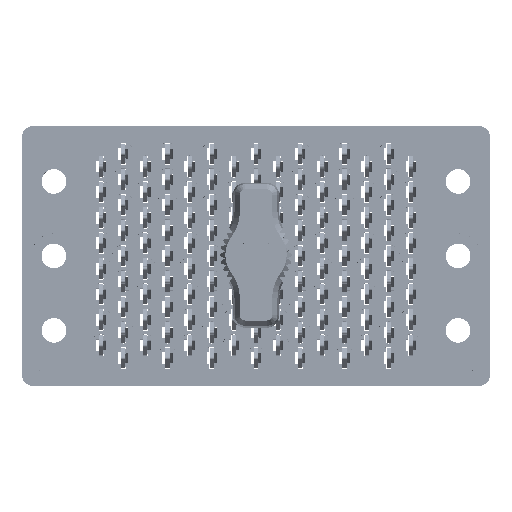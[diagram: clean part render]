
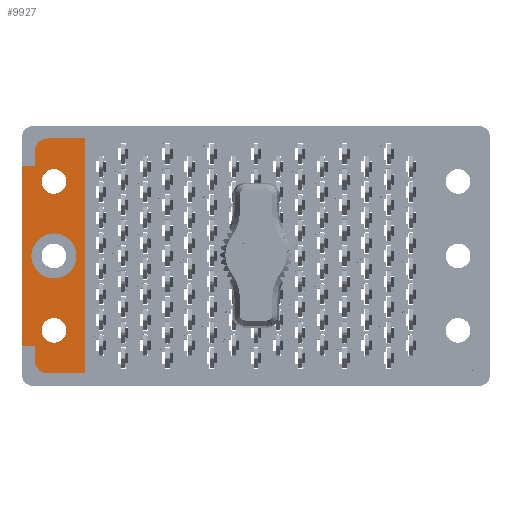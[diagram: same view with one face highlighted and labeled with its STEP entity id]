
A CAD part, top view. The second image highlights one B-rep face of the part: STEP entity #9927.
In plain terms, the highlighted planar face has unit normal (0, 0, 1).
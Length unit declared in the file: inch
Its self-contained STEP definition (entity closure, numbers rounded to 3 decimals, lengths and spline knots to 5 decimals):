
#209 = VERTEX_POINT ( 'NONE', #38791 ) ;
#692 = LINE ( 'NONE', #48378, #39513 ) ;
#1297 = AXIS2_PLACEMENT_3D ( 'NONE', #1905, #43440, #85039 ) ;
#1304 = ORIENTED_EDGE ( 'NONE', *, *, #89556, .T. ) ;
#1559 = ORIENTED_EDGE ( 'NONE', *, *, #34092, .T. ) ;
#1905 = CARTESIAN_POINT ( 'NONE',  ( -1.225, -0.615, -0.117 ) ) ;
#2947 = CARTESIAN_POINT ( 'NONE',  ( -1.3, -0.615, -0.117 ) ) ;
#5914 = EDGE_CURVE ( 'NONE', #89757, #19831, #66030, .T. ) ;
#6220 = CARTESIAN_POINT ( 'NONE',  ( -1.115, -0.4375, -0.117 ) ) ;
#6446 = EDGE_LOOP ( 'NONE', ( #1304, #7442, #56029, #1559, #35537, #18134, #103705, #23668, #94515, #49916 ) ) ;
#6774 = CIRCLE ( 'NONE', #94406, 0.1325 ) ;
#7442 = ORIENTED_EDGE ( 'NONE', *, *, #64470, .T. ) ;
#7954 = AXIS2_PLACEMENT_3D ( 'NONE', #32287, #89775, #40259 ) ;
#9914 = VERTEX_POINT ( 'NONE', #19978 ) ;
#9927 = ADVANCED_FACE ( 'NONE', ( #21981, #42694, #64714, #100878 ), #45953, .T. ) ;
#10055 = CIRCLE ( 'NONE', #101350, 0.0725 ) ;
#11209 = CARTESIAN_POINT ( 'NONE',  ( -1.1875, 0.4375, -0.117 ) ) ;
#11278 = CARTESIAN_POINT ( 'NONE',  ( -1.375, 0.7625, -0.117 ) ) ;
#11586 = AXIS2_PLACEMENT_3D ( 'NONE', #47549, #63877, #30263 ) ;
#11834 = EDGE_CURVE ( 'NONE', #74896, #93071, #10055, .T. ) ;
#13340 = DIRECTION ( 'NONE',  ( 0., -1., 0. ) ) ;
#13692 = CARTESIAN_POINT ( 'NONE',  ( -1.3, 0., -0.117 ) ) ;
#13851 = EDGE_CURVE ( 'NONE', #74258, #98178, #73009, .T. ) ;
#16038 = CARTESIAN_POINT ( 'NONE',  ( -1.26, -0.4375, -0.117 ) ) ;
#16805 = CARTESIAN_POINT ( 'NONE',  ( -1.375, -0.5285, -0.117 ) ) ;
#18134 = ORIENTED_EDGE ( 'NONE', *, *, #13851, .F. ) ;
#19831 = VERTEX_POINT ( 'NONE', #63570 ) ;
#19978 = CARTESIAN_POINT ( 'NONE',  ( -1.225, -0.69, -0.117 ) ) ;
#19990 = VERTEX_POINT ( 'NONE', #65697 ) ;
#20394 = DIRECTION ( 'NONE',  ( 0., 0., 1. ) ) ;
#21706 = AXIS2_PLACEMENT_3D ( 'NONE', #104197, #20394, #78242 ) ;
#21981 = FACE_BOUND ( 'NONE', #50403, .T. ) ;
#22866 = CARTESIAN_POINT ( 'NONE',  ( -1.1875, 0.4375, -0.117 ) ) ;
#22868 = DIRECTION ( 'NONE',  ( -1., 0., 0. ) ) ;
#23668 = ORIENTED_EDGE ( 'NONE', *, *, #26270, .T. ) ;
#25333 = ORIENTED_EDGE ( 'NONE', *, *, #78376, .F. ) ;
#26270 = EDGE_CURVE ( 'NONE', #56380, #9914, #60533, .T. ) ;
#28256 = EDGE_CURVE ( 'NONE', #19990, #98178, #93701, .T. ) ;
#28682 = CARTESIAN_POINT ( 'NONE',  ( -1.3, 0.5285, -0.117 ) ) ;
#30263 = DIRECTION ( 'NONE',  ( 1., 0., 0. ) ) ;
#30820 = DIRECTION ( 'NONE',  ( 0., 0., 1. ) ) ;
#31209 = CARTESIAN_POINT ( 'NONE',  ( -1.375, -0.7625, -0.117 ) ) ;
#32287 = CARTESIAN_POINT ( 'NONE',  ( -1.1875, -0.4375, -0.117 ) ) ;
#32443 = CARTESIAN_POINT ( 'NONE',  ( -1.3, 0., -0.117 ) ) ;
#32887 = ORIENTED_EDGE ( 'NONE', *, *, #11834, .F. ) ;
#34092 = EDGE_CURVE ( 'NONE', #68366, #19990, #69681, .T. ) ;
#35537 = ORIENTED_EDGE ( 'NONE', *, *, #28256, .T. ) ;
#35961 = VECTOR ( 'NONE', #13340, 39.37008 ) ;
#36409 = EDGE_CURVE ( 'NONE', #71787, #42363, #692, .T. ) ;
#38118 = CARTESIAN_POINT ( 'NONE',  ( -1.225, 0.69, -0.117 ) ) ;
#38159 = EDGE_LOOP ( 'NONE', ( #32887, #78122 ) ) ;
#38791 = CARTESIAN_POINT ( 'NONE',  ( -1.3, 0.615, -0.117 ) ) ;
#39125 = DIRECTION ( 'NONE',  ( 1., 0., 0. ) ) ;
#39513 = VECTOR ( 'NONE', #106195, 39.37008 ) ;
#39544 = DIRECTION ( 'NONE',  ( 0., 0., 1. ) ) ;
#40259 = DIRECTION ( 'NONE',  ( 1., 0., 0. ) ) ;
#41494 = EDGE_CURVE ( 'NONE', #104215, #96954, #6774, .T. ) ;
#42363 = VERTEX_POINT ( 'NONE', #54551 ) ;
#42694 = FACE_BOUND ( 'NONE', #38159, .T. ) ;
#42939 = DIRECTION ( 'NONE',  ( 1., 0., 0. ) ) ;
#43440 = DIRECTION ( 'NONE',  ( 0., 0., 1. ) ) ;
#44375 = CARTESIAN_POINT ( 'NONE',  ( -1.32, 0., -0.117 ) ) ;
#45236 = LINE ( 'NONE', #79374, #68521 ) ;
#45794 = CIRCLE ( 'NONE', #79547, 0.0725 ) ;
#45953 = PLANE ( 'NONE',  #94662 ) ;
#47549 = CARTESIAN_POINT ( 'NONE',  ( -1.1875, 0., -0.117 ) ) ;
#48051 = DIRECTION ( 'NONE',  ( -1., 0., 0. ) ) ;
#48378 = CARTESIAN_POINT ( 'NONE',  ( -1.005, 0.7625, -0.117 ) ) ;
#49248 = DIRECTION ( 'NONE',  ( 1., 0., 0. ) ) ;
#49916 = ORIENTED_EDGE ( 'NONE', *, *, #36409, .T. ) ;
#50403 = EDGE_LOOP ( 'NONE', ( #76034, #70587 ) ) ;
#51542 = EDGE_CURVE ( 'NONE', #71787, #9914, #45236, .T. ) ;
#53465 = LINE ( 'NONE', #32443, #80653 ) ;
#54051 = DIRECTION ( 'NONE',  ( -1., 0., 0. ) ) ;
#54426 = EDGE_CURVE ( 'NONE', #74258, #56380, #53465, .T. ) ;
#54551 = CARTESIAN_POINT ( 'NONE',  ( -1.005, 0.69, -0.117 ) ) ;
#55100 = CARTESIAN_POINT ( 'NONE',  ( -1.055, 0., -0.117 ) ) ;
#56029 = ORIENTED_EDGE ( 'NONE', *, *, #91668, .T. ) ;
#56380 = VERTEX_POINT ( 'NONE', #2947 ) ;
#57288 = ORIENTED_EDGE ( 'NONE', *, *, #41494, .F. ) ;
#57442 = CARTESIAN_POINT ( 'NONE',  ( 0., 0.69, -0.117 ) ) ;
#58260 = EDGE_CURVE ( 'NONE', #19831, #89757, #45794, .T. ) ;
#58478 = LINE ( 'NONE', #57442, #59731 ) ;
#58541 = CIRCLE ( 'NONE', #11586, 0.1325 ) ;
#59731 = VECTOR ( 'NONE', #90663, 39.37008 ) ;
#60533 = CIRCLE ( 'NONE', #1297, 0.075 ) ;
#61473 = CIRCLE ( 'NONE', #7954, 0.0725 ) ;
#63570 = CARTESIAN_POINT ( 'NONE',  ( -1.115, 0.4375, -0.117 ) ) ;
#63877 = DIRECTION ( 'NONE',  ( 0., 0., 1. ) ) ;
#64383 = LINE ( 'NONE', #13692, #35961 ) ;
#64470 = EDGE_CURVE ( 'NONE', #96852, #209, #67944, .T. ) ;
#64714 = FACE_BOUND ( 'NONE', #106373, .T. ) ;
#65528 = CARTESIAN_POINT ( 'NONE',  ( -1.005, -0.69, -0.117 ) ) ;
#65697 = CARTESIAN_POINT ( 'NONE',  ( -1.375, 0.5285, -0.117 ) ) ;
#66030 = CIRCLE ( 'NONE', #79137, 0.0725 ) ;
#67073 = VECTOR ( 'NONE', #48051, 39.37008 ) ;
#67468 = CARTESIAN_POINT ( 'NONE',  ( -1.1875, 0., -0.117 ) ) ;
#67511 = CARTESIAN_POINT ( 'NONE',  ( -1.26, 0.4375, -0.117 ) ) ;
#67827 = DIRECTION ( 'NONE',  ( 0., 0., 1. ) ) ;
#67944 = CIRCLE ( 'NONE', #21706, 0.075 ) ;
#68366 = VERTEX_POINT ( 'NONE', #28682 ) ;
#68521 = VECTOR ( 'NONE', #54051, 39.37008 ) ;
#69681 = LINE ( 'NONE', #105877, #67073 ) ;
#70587 = ORIENTED_EDGE ( 'NONE', *, *, #58260, .F. ) ;
#71787 = VERTEX_POINT ( 'NONE', #65528 ) ;
#73009 = LINE ( 'NONE', #73066, #92417 ) ;
#73021 = VECTOR ( 'NONE', #77455, 39.37008 ) ;
#73066 = CARTESIAN_POINT ( 'NONE',  ( 0., -0.5285, -0.117 ) ) ;
#74258 = VERTEX_POINT ( 'NONE', #74719 ) ;
#74719 = CARTESIAN_POINT ( 'NONE',  ( -1.3, -0.5285, -0.117 ) ) ;
#74896 = VERTEX_POINT ( 'NONE', #16038 ) ;
#75492 = DIRECTION ( 'NONE',  ( 0., 0., 1. ) ) ;
#75860 = CARTESIAN_POINT ( 'NONE',  ( -1.1875, -0.4375, -0.117 ) ) ;
#76034 = ORIENTED_EDGE ( 'NONE', *, *, #5914, .F. ) ;
#77455 = DIRECTION ( 'NONE',  ( 0., -1., 0. ) ) ;
#78115 = DIRECTION ( 'NONE',  ( 0., 0., 1. ) ) ;
#78122 = ORIENTED_EDGE ( 'NONE', *, *, #86723, .F. ) ;
#78242 = DIRECTION ( 'NONE',  ( 1., 0., 0. ) ) ;
#78376 = EDGE_CURVE ( 'NONE', #96954, #104215, #58541, .T. ) ;
#79137 = AXIS2_PLACEMENT_3D ( 'NONE', #22866, #30820, #39125 ) ;
#79374 = CARTESIAN_POINT ( 'NONE',  ( 0., -0.69, -0.117 ) ) ;
#79547 = AXIS2_PLACEMENT_3D ( 'NONE', #11209, #78115, #86381 ) ;
#80653 = VECTOR ( 'NONE', #81984, 39.37008 ) ;
#81984 = DIRECTION ( 'NONE',  ( 0., -1., 0. ) ) ;
#84106 = DIRECTION ( 'NONE',  ( 1., 0., 0. ) ) ;
#85039 = DIRECTION ( 'NONE',  ( 1., 0., 0. ) ) ;
#86381 = DIRECTION ( 'NONE',  ( 1., 0., 0. ) ) ;
#86723 = EDGE_CURVE ( 'NONE', #93071, #74896, #61473, .T. ) ;
#89556 = EDGE_CURVE ( 'NONE', #42363, #96852, #58478, .T. ) ;
#89757 = VERTEX_POINT ( 'NONE', #67511 ) ;
#89775 = DIRECTION ( 'NONE',  ( 0., 0., 1. ) ) ;
#90663 = DIRECTION ( 'NONE',  ( -1., 0., 0. ) ) ;
#91668 = EDGE_CURVE ( 'NONE', #209, #68366, #64383, .T. ) ;
#92417 = VECTOR ( 'NONE', #22868, 39.37008 ) ;
#93071 = VERTEX_POINT ( 'NONE', #6220 ) ;
#93701 = LINE ( 'NONE', #11278, #73021 ) ;
#94406 = AXIS2_PLACEMENT_3D ( 'NONE', #67468, #67827, #84106 ) ;
#94515 = ORIENTED_EDGE ( 'NONE', *, *, #51542, .F. ) ;
#94662 = AXIS2_PLACEMENT_3D ( 'NONE', #31209, #39544, #49248 ) ;
#96852 = VERTEX_POINT ( 'NONE', #38118 ) ;
#96954 = VERTEX_POINT ( 'NONE', #55100 ) ;
#98178 = VERTEX_POINT ( 'NONE', #16805 ) ;
#100878 = FACE_OUTER_BOUND ( 'NONE', #6446, .T. ) ;
#101350 = AXIS2_PLACEMENT_3D ( 'NONE', #75860, #75492, #42939 ) ;
#103705 = ORIENTED_EDGE ( 'NONE', *, *, #54426, .T. ) ;
#104197 = CARTESIAN_POINT ( 'NONE',  ( -1.225, 0.615, -0.117 ) ) ;
#104215 = VERTEX_POINT ( 'NONE', #44375 ) ;
#105877 = CARTESIAN_POINT ( 'NONE',  ( 0., 0.5285, -0.117 ) ) ;
#106195 = DIRECTION ( 'NONE',  ( 0., 1., 0. ) ) ;
#106373 = EDGE_LOOP ( 'NONE', ( #25333, #57288 ) ) ;
